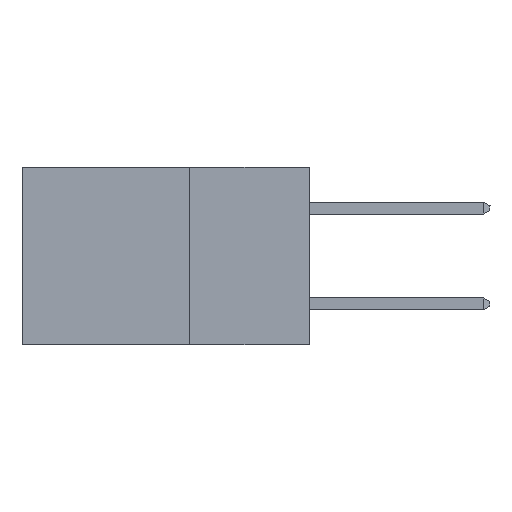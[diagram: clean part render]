
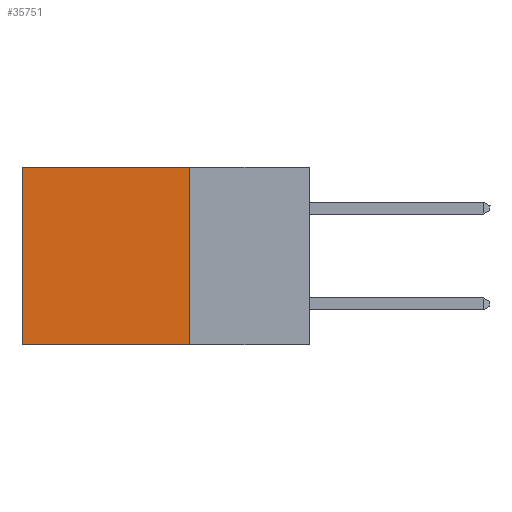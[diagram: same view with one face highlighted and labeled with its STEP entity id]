
A CAD part, left-side view. The second image highlights one B-rep face of the part: STEP entity #35751.
In plain terms, the highlighted planar face has unit normal (-1, 0, 0).
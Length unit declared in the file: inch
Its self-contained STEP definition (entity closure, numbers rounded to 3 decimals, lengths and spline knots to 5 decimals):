
#1455 = DIRECTION ( 'NONE',  ( 0., 0., -1. ) ) ;
#1600 = EDGE_CURVE ( 'NONE', #5600, #27526, #37053, .T. ) ;
#2643 = CARTESIAN_POINT ( 'NONE',  ( 0.2875, 0.25, 0. ) ) ;
#2878 = VERTEX_POINT ( 'NONE', #2643 ) ;
#3411 = DIRECTION ( 'NONE',  ( 0., 1., 0. ) ) ;
#4334 = VECTOR ( 'NONE', #37272, 39.37008 ) ;
#5600 = VERTEX_POINT ( 'NONE', #23551 ) ;
#5967 = CARTESIAN_POINT ( 'NONE',  ( 0.2875, 0.6, -0.37 ) ) ;
#7218 = CARTESIAN_POINT ( 'NONE',  ( 0.2875, 0.6, 0. ) ) ;
#7484 = EDGE_CURVE ( 'NONE', #2878, #9202, #13482, .T. ) ;
#9202 = VERTEX_POINT ( 'NONE', #7218 ) ;
#9870 = DIRECTION ( 'NONE',  ( 1., 0., 0. ) ) ;
#10394 = CARTESIAN_POINT ( 'NONE',  ( 0.2875, 0.25, 0. ) ) ;
#13482 = LINE ( 'NONE', #31010, #4334 ) ;
#15392 = AXIS2_PLACEMENT_3D ( 'NONE', #10394, #9870, #37686 ) ;
#15618 = CARTESIAN_POINT ( 'NONE',  ( 0.2875, 0.25, -0.37 ) ) ;
#15704 = ORIENTED_EDGE ( 'NONE', *, *, #18988, .F. ) ;
#18988 = EDGE_CURVE ( 'NONE', #2878, #5600, #39332, .T. ) ;
#20758 = VECTOR ( 'NONE', #1455, 39.37008 ) ;
#20958 = ORIENTED_EDGE ( 'NONE', *, *, #36869, .T. ) ;
#21570 = EDGE_LOOP ( 'NONE', ( #20958, #26760, #15704, #27500 ) ) ;
#23551 = CARTESIAN_POINT ( 'NONE',  ( 0.2875, 0.25, -0.37 ) ) ;
#25728 = PLANE ( 'NONE',  #15392 ) ;
#26067 = CARTESIAN_POINT ( 'NONE',  ( 0.2875, 0.6, 0. ) ) ;
#26167 = VECTOR ( 'NONE', #27147, 39.37008 ) ;
#26760 = ORIENTED_EDGE ( 'NONE', *, *, #1600, .F. ) ;
#27147 = DIRECTION ( 'NONE',  ( 0., 0., -1. ) ) ;
#27500 = ORIENTED_EDGE ( 'NONE', *, *, #7484, .T. ) ;
#27526 = VERTEX_POINT ( 'NONE', #5967 ) ;
#28815 = VECTOR ( 'NONE', #3411, 39.37008 ) ;
#30933 = LINE ( 'NONE', #26067, #20758 ) ;
#31010 = CARTESIAN_POINT ( 'NONE',  ( 0.2875, 0.25, 0. ) ) ;
#35751 = ADVANCED_FACE ( 'NONE', ( #39740 ), #25728, .F. ) ;
#36776 = CARTESIAN_POINT ( 'NONE',  ( 0.2875, 0.25, 0. ) ) ;
#36869 = EDGE_CURVE ( 'NONE', #9202, #27526, #30933, .T. ) ;
#37053 = LINE ( 'NONE', #15618, #28815 ) ;
#37272 = DIRECTION ( 'NONE',  ( 0., 1., 0. ) ) ;
#37686 = DIRECTION ( 'NONE',  ( 0., 0., -1. ) ) ;
#39332 = LINE ( 'NONE', #36776, #26167 ) ;
#39740 = FACE_OUTER_BOUND ( 'NONE', #21570, .T. ) ;
